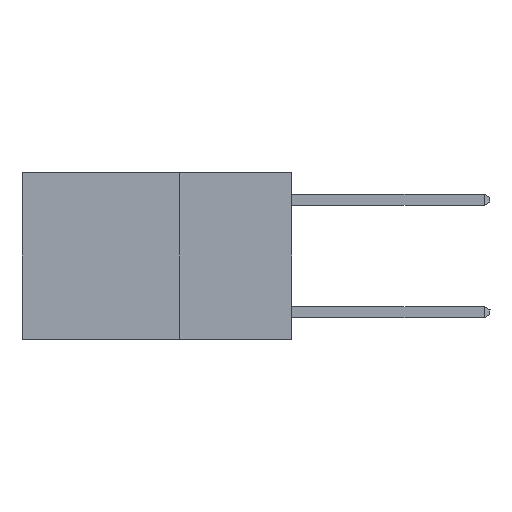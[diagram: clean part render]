
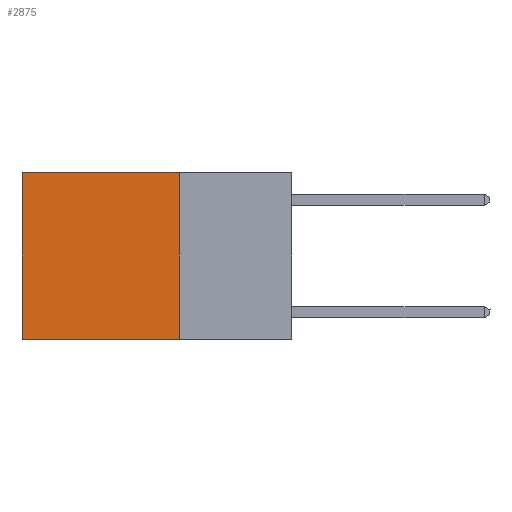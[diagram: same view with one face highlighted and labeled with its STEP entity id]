
A CAD part, left-side view. The second image highlights one B-rep face of the part: STEP entity #2875.
In plain terms, the highlighted planar face has unit normal (-1, 0, 0).
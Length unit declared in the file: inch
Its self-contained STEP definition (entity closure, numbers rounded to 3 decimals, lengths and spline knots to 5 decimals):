
#269 = DIRECTION ( 'NONE',  ( 0., 0., -1. ) ) ;
#272 = EDGE_CURVE ( 'NONE', #3821, #2817, #2298, .T. ) ;
#353 = LINE ( 'NONE', #3211, #7799 ) ;
#404 = VECTOR ( 'NONE', #4992, 39.37008 ) ;
#544 = ORIENTED_EDGE ( 'NONE', *, *, #6549, .T. ) ;
#767 = LINE ( 'NONE', #4281, #4508 ) ;
#2118 = EDGE_LOOP ( 'NONE', ( #544, #2460, #6345, #2709 ) ) ;
#2294 = DIRECTION ( 'NONE',  ( 0., 0., -1. ) ) ;
#2298 = LINE ( 'NONE', #8562, #404 ) ;
#2460 = ORIENTED_EDGE ( 'NONE', *, *, #272, .F. ) ;
#2709 = ORIENTED_EDGE ( 'NONE', *, *, #8729, .T. ) ;
#2817 = VERTEX_POINT ( 'NONE', #8689 ) ;
#2875 = ADVANCED_FACE ( 'NONE', ( #7481 ), #6248, .F. ) ;
#3077 = DIRECTION ( 'NONE',  ( 0., 0., -1. ) ) ;
#3211 = CARTESIAN_POINT ( 'NONE',  ( 0.2625, 0.6, 0. ) ) ;
#3821 = VERTEX_POINT ( 'NONE', #6033 ) ;
#3885 = CARTESIAN_POINT ( 'NONE',  ( 0.2625, 0.25, 0. ) ) ;
#4064 = VECTOR ( 'NONE', #2294, 39.37008 ) ;
#4281 = CARTESIAN_POINT ( 'NONE',  ( 0.2625, 0.25, 0. ) ) ;
#4508 = VECTOR ( 'NONE', #7767, 39.37008 ) ;
#4992 = DIRECTION ( 'NONE',  ( 0., 1., 0. ) ) ;
#5244 = DIRECTION ( 'NONE',  ( 1., 0., 0. ) ) ;
#5468 = CARTESIAN_POINT ( 'NONE',  ( 0.2625, 0.25, 0. ) ) ;
#5768 = VERTEX_POINT ( 'NONE', #5468 ) ;
#5903 = LINE ( 'NONE', #5962, #4064 ) ;
#5962 = CARTESIAN_POINT ( 'NONE',  ( 0.2625, 0.25, 0. ) ) ;
#6033 = CARTESIAN_POINT ( 'NONE',  ( 0.2625, 0.25, -0.37 ) ) ;
#6148 = CARTESIAN_POINT ( 'NONE',  ( 0.2625, 0.6, 0. ) ) ;
#6248 = PLANE ( 'NONE',  #8666 ) ;
#6345 = ORIENTED_EDGE ( 'NONE', *, *, #8235, .F. ) ;
#6549 = EDGE_CURVE ( 'NONE', #9309, #2817, #353, .T. ) ;
#7481 = FACE_OUTER_BOUND ( 'NONE', #2118, .T. ) ;
#7767 = DIRECTION ( 'NONE',  ( 0., 1., 0. ) ) ;
#7799 = VECTOR ( 'NONE', #269, 39.37008 ) ;
#8235 = EDGE_CURVE ( 'NONE', #5768, #3821, #5903, .T. ) ;
#8562 = CARTESIAN_POINT ( 'NONE',  ( 0.2625, 0.25, -0.37 ) ) ;
#8666 = AXIS2_PLACEMENT_3D ( 'NONE', #3885, #5244, #3077 ) ;
#8689 = CARTESIAN_POINT ( 'NONE',  ( 0.2625, 0.6, -0.37 ) ) ;
#8729 = EDGE_CURVE ( 'NONE', #5768, #9309, #767, .T. ) ;
#9309 = VERTEX_POINT ( 'NONE', #6148 ) ;
